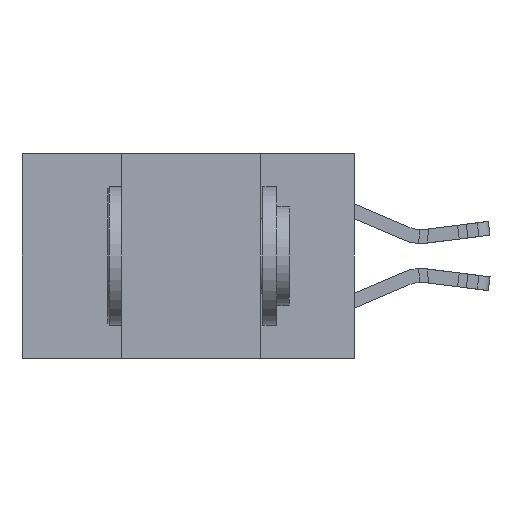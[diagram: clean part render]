
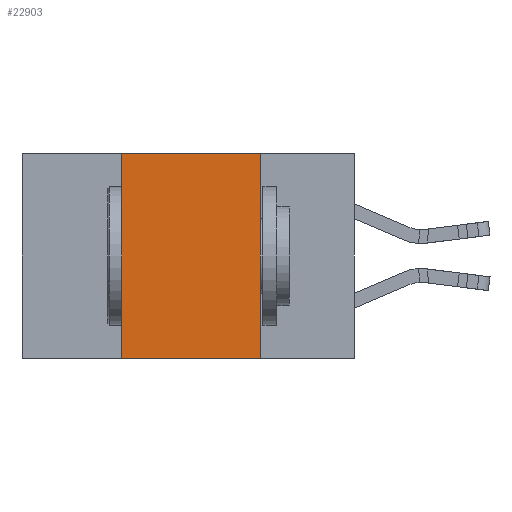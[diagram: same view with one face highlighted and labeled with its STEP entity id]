
A CAD part, left-side view. The second image highlights one B-rep face of the part: STEP entity #22903.
In plain terms, the highlighted planar face has unit normal (-1, 0, 0).
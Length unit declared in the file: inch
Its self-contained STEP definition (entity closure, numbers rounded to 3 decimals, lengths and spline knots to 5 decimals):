
#825 = VERTEX_POINT ( 'NONE', #31798 ) ;
#1426 = CARTESIAN_POINT ( 'NONE',  ( 0., 0.6, 0. ) ) ;
#2696 = VECTOR ( 'NONE', #6697, 39.37008 ) ;
#5399 = FACE_OUTER_BOUND ( 'NONE', #9231, .T. ) ;
#6111 = CARTESIAN_POINT ( 'NONE',  ( 0., 0.17, 0. ) ) ;
#6697 = DIRECTION ( 'NONE',  ( 0., 0., 1. ) ) ;
#6766 = DIRECTION ( 'NONE',  ( 0., -1., 0. ) ) ;
#7545 = EDGE_CURVE ( 'NONE', #31828, #825, #19019, .T. ) ;
#8201 = DIRECTION ( 'NONE',  ( 1., 0., 0. ) ) ;
#9231 = EDGE_LOOP ( 'NONE', ( #13444, #19492, #21518, #23304 ) ) ;
#10924 = PLANE ( 'NONE',  #29883 ) ;
#11771 = DIRECTION ( 'NONE',  ( 0., -1., 0. ) ) ;
#11994 = CARTESIAN_POINT ( 'NONE',  ( 0., 0.6, -0.37 ) ) ;
#13444 = ORIENTED_EDGE ( 'NONE', *, *, #24135, .F. ) ;
#14878 = CARTESIAN_POINT ( 'NONE',  ( 0., 0.42, 0. ) ) ;
#14948 = CARTESIAN_POINT ( 'NONE',  ( 0., 0.17, 0. ) ) ;
#16994 = VERTEX_POINT ( 'NONE', #6111 ) ;
#17896 = LINE ( 'NONE', #11994, #19890 ) ;
#19019 = LINE ( 'NONE', #14878, #2696 ) ;
#19492 = ORIENTED_EDGE ( 'NONE', *, *, #28857, .F. ) ;
#19890 = VECTOR ( 'NONE', #11771, 39.37008 ) ;
#21196 = CARTESIAN_POINT ( 'NONE',  ( 0., 0.6, 0. ) ) ;
#21518 = ORIENTED_EDGE ( 'NONE', *, *, #7545, .F. ) ;
#22342 = VECTOR ( 'NONE', #6766, 39.37008 ) ;
#22849 = LINE ( 'NONE', #14948, #28133 ) ;
#22903 = ADVANCED_FACE ( 'NONE', ( #5399 ), #10924, .F. ) ;
#23304 = ORIENTED_EDGE ( 'NONE', *, *, #28888, .T. ) ;
#24135 = EDGE_CURVE ( 'NONE', #16994, #29084, #22849, .T. ) ;
#28133 = VECTOR ( 'NONE', #28497, 39.37008 ) ;
#28497 = DIRECTION ( 'NONE',  ( 0., 0., -1. ) ) ;
#28857 = EDGE_CURVE ( 'NONE', #825, #16994, #31680, .T. ) ;
#28888 = EDGE_CURVE ( 'NONE', #31828, #29084, #17896, .T. ) ;
#29084 = VERTEX_POINT ( 'NONE', #33493 ) ;
#29883 = AXIS2_PLACEMENT_3D ( 'NONE', #21196, #8201, #31296 ) ;
#29885 = CARTESIAN_POINT ( 'NONE',  ( 0., 0.42, -0.37 ) ) ;
#31296 = DIRECTION ( 'NONE',  ( 0., 0., -1. ) ) ;
#31680 = LINE ( 'NONE', #1426, #22342 ) ;
#31798 = CARTESIAN_POINT ( 'NONE',  ( 0., 0.42, 0. ) ) ;
#31828 = VERTEX_POINT ( 'NONE', #29885 ) ;
#33493 = CARTESIAN_POINT ( 'NONE',  ( 0., 0.17, -0.37 ) ) ;
